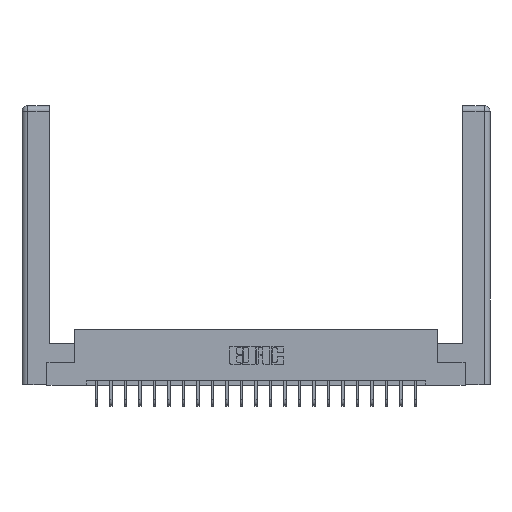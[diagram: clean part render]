
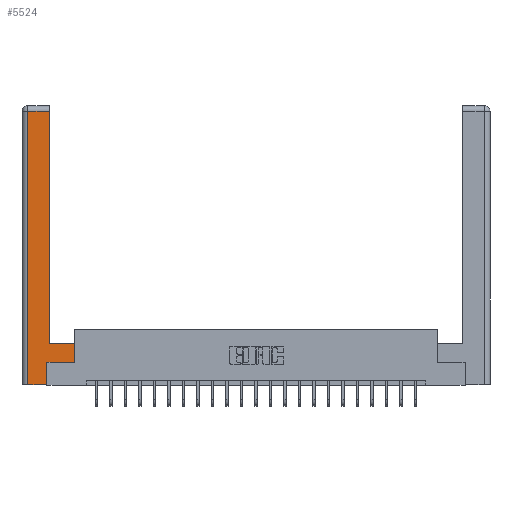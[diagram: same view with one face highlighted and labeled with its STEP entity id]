
A CAD part, top view. The second image highlights one B-rep face of the part: STEP entity #5524.
In plain terms, the highlighted planar face has unit normal (0, 0, 1).
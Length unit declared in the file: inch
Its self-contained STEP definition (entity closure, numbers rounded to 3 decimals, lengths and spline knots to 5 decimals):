
#1016 = CARTESIAN_POINT ( 'NONE',  ( 0.565, 0.245, 0. ) ) ;
#1062 = ORIENTED_EDGE ( 'NONE', *, *, #20112, .T. ) ;
#1113 = LINE ( 'NONE', #23363, #2294 ) ;
#1324 = DIRECTION ( 'NONE',  ( 0., 1., 0. ) ) ;
#2294 = VECTOR ( 'NONE', #19665, 39.37008 ) ;
#2477 = CARTESIAN_POINT ( 'NONE',  ( 0.0615, 2.94, 0. ) ) ;
#2612 = ORIENTED_EDGE ( 'NONE', *, *, #14149, .T. ) ;
#2800 = VERTEX_POINT ( 'NONE', #8272 ) ;
#2817 = VECTOR ( 'NONE', #17025, 39.37008 ) ;
#4187 = CARTESIAN_POINT ( 'NONE',  ( 0.265, 0.245, 0. ) ) ;
#4295 = VERTEX_POINT ( 'NONE', #22967 ) ;
#4819 = DIRECTION ( 'NONE',  ( -1., 0., 0. ) ) ;
#4878 = CARTESIAN_POINT ( 'NONE',  ( 0.565, 0.45, 0. ) ) ;
#4983 = CARTESIAN_POINT ( 'NONE',  ( 0.295, 0.45, 0. ) ) ;
#5240 = VECTOR ( 'NONE', #1324, 39.37008 ) ;
#5282 = LINE ( 'NONE', #23277, #8602 ) ;
#5524 = ADVANCED_FACE ( 'NONE', ( #18523 ), #15023, .F. ) ;
#6087 = ORIENTED_EDGE ( 'NONE', *, *, #13910, .T. ) ;
#6400 = CARTESIAN_POINT ( 'NONE',  ( 0.295, 3., 0. ) ) ;
#6567 = DIRECTION ( 'NONE',  ( 0., 1., 0. ) ) ;
#6899 = CARTESIAN_POINT ( 'NONE',  ( 0.0615, 0., 0. ) ) ;
#8272 = CARTESIAN_POINT ( 'NONE',  ( 0.295, 2.94, 0. ) ) ;
#8602 = VECTOR ( 'NONE', #15796, 39.37008 ) ;
#8875 = LINE ( 'NONE', #6899, #9149 ) ;
#9071 = DIRECTION ( 'NONE',  ( 0., 1., 0. ) ) ;
#9149 = VECTOR ( 'NONE', #20325, 39.37008 ) ;
#10059 = VERTEX_POINT ( 'NONE', #4878 ) ;
#10223 = ORIENTED_EDGE ( 'NONE', *, *, #12246, .T. ) ;
#10568 = VERTEX_POINT ( 'NONE', #1016 ) ;
#11104 = ORIENTED_EDGE ( 'NONE', *, *, #22387, .T. ) ;
#11279 = LINE ( 'NONE', #23752, #12509 ) ;
#12246 = EDGE_CURVE ( 'NONE', #13358, #10568, #18980, .T. ) ;
#12509 = VECTOR ( 'NONE', #4819, 39.37008 ) ;
#12672 = VERTEX_POINT ( 'NONE', #4983 ) ;
#12792 = CARTESIAN_POINT ( 'NONE',  ( 0.565, 0.45, 0. ) ) ;
#12915 = ORIENTED_EDGE ( 'NONE', *, *, #14165, .T. ) ;
#13110 = AXIS2_PLACEMENT_3D ( 'NONE', #14938, #15514, #21207 ) ;
#13187 = CARTESIAN_POINT ( 'NONE',  ( 0.265, 0.245, 0. ) ) ;
#13358 = VERTEX_POINT ( 'NONE', #4187 ) ;
#13910 = EDGE_CURVE ( 'NONE', #10059, #12672, #11279, .T. ) ;
#14149 = EDGE_CURVE ( 'NONE', #2800, #19093, #1113, .T. ) ;
#14165 = EDGE_CURVE ( 'NONE', #4295, #19034, #5282, .T. ) ;
#14938 = CARTESIAN_POINT ( 'NONE',  ( 0., 0., 0. ) ) ;
#14944 = LINE ( 'NONE', #13187, #16733 ) ;
#15023 = PLANE ( 'NONE',  #13110 ) ;
#15497 = CARTESIAN_POINT ( 'NONE',  ( 0.265, 0., 0. ) ) ;
#15514 = DIRECTION ( 'NONE',  ( 0., 0., -1. ) ) ;
#15731 = LINE ( 'NONE', #12792, #5240 ) ;
#15796 = DIRECTION ( 'NONE',  ( 1., 0., 0. ) ) ;
#16005 = EDGE_CURVE ( 'NONE', #12672, #2800, #21655, .T. ) ;
#16205 = EDGE_LOOP ( 'NONE', ( #21220, #2612, #1062, #12915, #19958, #10223, #11104, #6087 ) ) ;
#16243 = VECTOR ( 'NONE', #6567, 39.37008 ) ;
#16733 = VECTOR ( 'NONE', #9071, 39.37008 ) ;
#17025 = DIRECTION ( 'NONE',  ( 1., 0., 0. ) ) ;
#17663 = EDGE_CURVE ( 'NONE', #19034, #13358, #14944, .T. ) ;
#18215 = CARTESIAN_POINT ( 'NONE',  ( 0.565, 0.245, 0. ) ) ;
#18523 = FACE_OUTER_BOUND ( 'NONE', #16205, .T. ) ;
#18980 = LINE ( 'NONE', #18215, #2817 ) ;
#19034 = VERTEX_POINT ( 'NONE', #15497 ) ;
#19093 = VERTEX_POINT ( 'NONE', #2477 ) ;
#19665 = DIRECTION ( 'NONE',  ( -1., 0., 0. ) ) ;
#19958 = ORIENTED_EDGE ( 'NONE', *, *, #17663, .T. ) ;
#20112 = EDGE_CURVE ( 'NONE', #19093, #4295, #8875, .T. ) ;
#20325 = DIRECTION ( 'NONE',  ( 0., -1., 0. ) ) ;
#21207 = DIRECTION ( 'NONE',  ( -1., 0., 0. ) ) ;
#21220 = ORIENTED_EDGE ( 'NONE', *, *, #16005, .T. ) ;
#21655 = LINE ( 'NONE', #6400, #16243 ) ;
#22387 = EDGE_CURVE ( 'NONE', #10568, #10059, #15731, .T. ) ;
#22967 = CARTESIAN_POINT ( 'NONE',  ( 0.0615, 0., 0. ) ) ;
#23277 = CARTESIAN_POINT ( 'NONE',  ( 0.265, 0., 0. ) ) ;
#23363 = CARTESIAN_POINT ( 'NONE',  ( 0.0615, 2.94, 0. ) ) ;
#23752 = CARTESIAN_POINT ( 'NONE',  ( 0.295, 0.45, 0. ) ) ;
